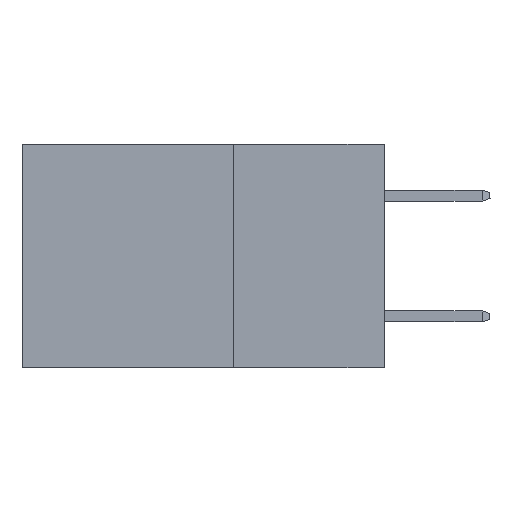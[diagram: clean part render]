
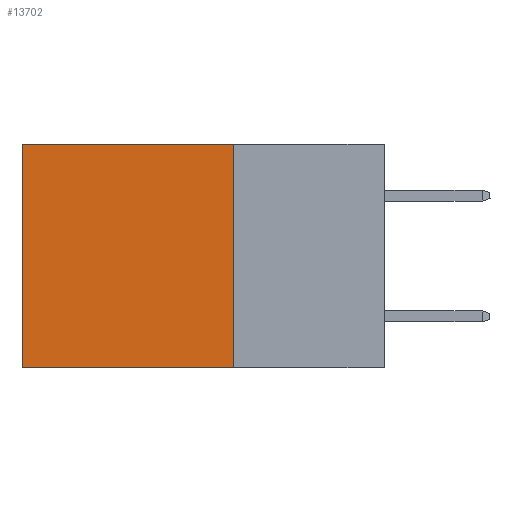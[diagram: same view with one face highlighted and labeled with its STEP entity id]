
A CAD part, left-side view. The second image highlights one B-rep face of the part: STEP entity #13702.
In plain terms, the highlighted planar face has unit normal (-1, 0, 0).
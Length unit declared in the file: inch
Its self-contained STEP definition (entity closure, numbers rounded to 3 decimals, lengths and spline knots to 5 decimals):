
#538 = VERTEX_POINT ( 'NONE', #24960 ) ;
#617 = CARTESIAN_POINT ( 'NONE',  ( 0.298, 0.25, -0.37 ) ) ;
#1162 = AXIS2_PLACEMENT_3D ( 'NONE', #18655, #8794, #22594 ) ;
#1894 = EDGE_CURVE ( 'NONE', #13760, #14065, #2306, .T. ) ;
#2136 = EDGE_LOOP ( 'NONE', ( #7914, #13571, #8796, #10542 ) ) ;
#2306 = LINE ( 'NONE', #9999, #16869 ) ;
#4315 = VECTOR ( 'NONE', #5559, 39.37008 ) ;
#4864 = VECTOR ( 'NONE', #16935, 39.37008 ) ;
#5243 = DIRECTION ( 'NONE',  ( 0., 0., -1. ) ) ;
#5559 = DIRECTION ( 'NONE',  ( 0., 1., 0. ) ) ;
#6661 = VECTOR ( 'NONE', #5243, 39.37008 ) ;
#7175 = CARTESIAN_POINT ( 'NONE',  ( 0.298, 0.25, 0. ) ) ;
#7914 = ORIENTED_EDGE ( 'NONE', *, *, #20003, .T. ) ;
#8794 = DIRECTION ( 'NONE',  ( 1., 0., 0. ) ) ;
#8796 = ORIENTED_EDGE ( 'NONE', *, *, #24958, .F. ) ;
#9999 = CARTESIAN_POINT ( 'NONE',  ( 0.298, 0.25, 0. ) ) ;
#10405 = EDGE_CURVE ( 'NONE', #18493, #538, #14252, .T. ) ;
#10542 = ORIENTED_EDGE ( 'NONE', *, *, #1894, .T. ) ;
#13144 = CARTESIAN_POINT ( 'NONE',  ( 0.298, 0.6, 0. ) ) ;
#13571 = ORIENTED_EDGE ( 'NONE', *, *, #10405, .F. ) ;
#13702 = ADVANCED_FACE ( 'NONE', ( #19601 ), #14708, .F. ) ;
#13760 = VERTEX_POINT ( 'NONE', #22766 ) ;
#14065 = VERTEX_POINT ( 'NONE', #25508 ) ;
#14252 = LINE ( 'NONE', #17404, #4315 ) ;
#14708 = PLANE ( 'NONE',  #1162 ) ;
#16869 = VECTOR ( 'NONE', #22719, 39.37008 ) ;
#16935 = DIRECTION ( 'NONE',  ( 0., 0., -1. ) ) ;
#17182 = LINE ( 'NONE', #13144, #6661 ) ;
#17404 = CARTESIAN_POINT ( 'NONE',  ( 0.298, 0.25, -0.37 ) ) ;
#17561 = LINE ( 'NONE', #7175, #4864 ) ;
#18493 = VERTEX_POINT ( 'NONE', #617 ) ;
#18655 = CARTESIAN_POINT ( 'NONE',  ( 0.298, 0.25, 0. ) ) ;
#19601 = FACE_OUTER_BOUND ( 'NONE', #2136, .T. ) ;
#20003 = EDGE_CURVE ( 'NONE', #14065, #538, #17182, .T. ) ;
#22594 = DIRECTION ( 'NONE',  ( 0., 0., -1. ) ) ;
#22719 = DIRECTION ( 'NONE',  ( 0., 1., 0. ) ) ;
#22766 = CARTESIAN_POINT ( 'NONE',  ( 0.298, 0.25, 0. ) ) ;
#24958 = EDGE_CURVE ( 'NONE', #13760, #18493, #17561, .T. ) ;
#24960 = CARTESIAN_POINT ( 'NONE',  ( 0.298, 0.6, -0.37 ) ) ;
#25508 = CARTESIAN_POINT ( 'NONE',  ( 0.298, 0.6, 0. ) ) ;
